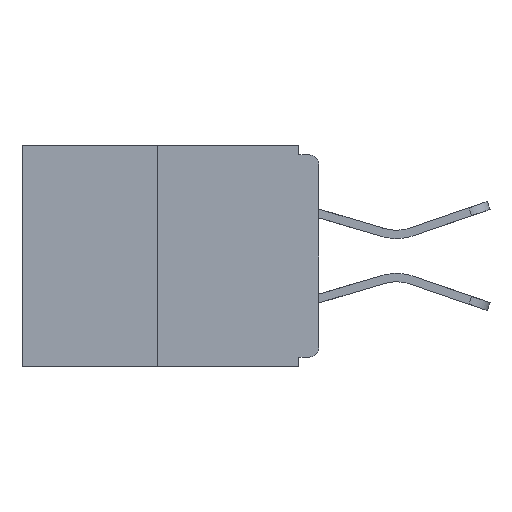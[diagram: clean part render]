
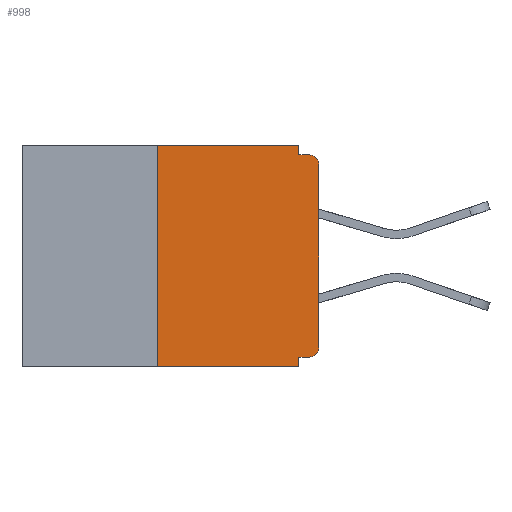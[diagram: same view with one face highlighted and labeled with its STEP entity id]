
A CAD part, left-side view. The second image highlights one B-rep face of the part: STEP entity #998.
In plain terms, the highlighted planar face has unit normal (-1, 0, 0).
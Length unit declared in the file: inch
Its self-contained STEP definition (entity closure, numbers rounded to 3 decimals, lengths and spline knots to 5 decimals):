
#89 = DIRECTION ( 'NONE',  ( 1., 0., 0. ) ) ;
#129 = DIRECTION ( 'NONE',  ( -1., 0., 0. ) ) ;
#150 = VERTEX_POINT ( 'NONE', #5514 ) ;
#182 = VECTOR ( 'NONE', #2445, 39.37008 ) ;
#286 = EDGE_CURVE ( 'NONE', #150, #296, #9862, .T. ) ;
#296 = VERTEX_POINT ( 'NONE', #3870 ) ;
#387 = AXIS2_PLACEMENT_3D ( 'NONE', #6551, #129, #1014 ) ;
#467 = CARTESIAN_POINT ( 'NONE',  ( 0., 0.031, -0.015 ) ) ;
#834 = ORIENTED_EDGE ( 'NONE', *, *, #11553, .T. ) ;
#934 = CARTESIAN_POINT ( 'NONE',  ( 0., 0., -0.015 ) ) ;
#998 = ADVANCED_FACE ( 'NONE', ( #4077 ), #4645, .F. ) ;
#1014 = DIRECTION ( 'NONE',  ( 0., 0., -1. ) ) ;
#1047 = LINE ( 'NONE', #1260, #4214 ) ;
#1260 = CARTESIAN_POINT ( 'NONE',  ( 0., 0., -0.328 ) ) ;
#1439 = DIRECTION ( 'NONE',  ( 0., -1., 0. ) ) ;
#1524 = CARTESIAN_POINT ( 'NONE',  ( 0., 0.25, 0. ) ) ;
#1578 = DIRECTION ( 'NONE',  ( 0., -1., 0. ) ) ;
#1853 = VERTEX_POINT ( 'NONE', #8227 ) ;
#2208 = LINE ( 'NONE', #5937, #7402 ) ;
#2445 = DIRECTION ( 'NONE',  ( 0., 0., 1. ) ) ;
#2594 = AXIS2_PLACEMENT_3D ( 'NONE', #10205, #89, #6673 ) ;
#2837 = ORIENTED_EDGE ( 'NONE', *, *, #9714, .T. ) ;
#3101 = EDGE_CURVE ( 'NONE', #1853, #10226, #9412, .T. ) ;
#3287 = DIRECTION ( 'NONE',  ( 0., 0., -1. ) ) ;
#3870 = CARTESIAN_POINT ( 'NONE',  ( 0., 0.031, -0.343 ) ) ;
#3915 = CARTESIAN_POINT ( 'NONE',  ( 0., 0., -0.313 ) ) ;
#3961 = CARTESIAN_POINT ( 'NONE',  ( 0., 0.015, -0.328 ) ) ;
#4077 = FACE_OUTER_BOUND ( 'NONE', #4302, .T. ) ;
#4214 = VECTOR ( 'NONE', #10363, 39.37008 ) ;
#4229 = DIRECTION ( 'NONE',  ( 0., 0., -1. ) ) ;
#4302 = EDGE_LOOP ( 'NONE', ( #8157, #7699, #10369, #8915, #7518, #834, #2837, #8779, #9005, #10305 ) ) ;
#4442 = CARTESIAN_POINT ( 'NONE',  ( 0., 0., -0.03 ) ) ;
#4645 = PLANE ( 'NONE',  #2594 ) ;
#4721 = EDGE_CURVE ( 'NONE', #1853, #296, #9951, .T. ) ;
#4926 = VERTEX_POINT ( 'NONE', #3961 ) ;
#4972 = AXIS2_PLACEMENT_3D ( 'NONE', #11584, #9837, #3287 ) ;
#5293 = CARTESIAN_POINT ( 'NONE',  ( 0., 0.46, -0.343 ) ) ;
#5315 = EDGE_CURVE ( 'NONE', #11823, #6057, #11917, .T. ) ;
#5514 = CARTESIAN_POINT ( 'NONE',  ( 0., 0.031, -0.328 ) ) ;
#5564 = CARTESIAN_POINT ( 'NONE',  ( 0., 0.015, -0.015 ) ) ;
#5712 = CARTESIAN_POINT ( 'NONE',  ( 0., 0., 0. ) ) ;
#5937 = CARTESIAN_POINT ( 'NONE',  ( 0., 0.031, 0. ) ) ;
#6057 = VERTEX_POINT ( 'NONE', #5564 ) ;
#6310 = EDGE_CURVE ( 'NONE', #11506, #6057, #7769, .T. ) ;
#6551 = CARTESIAN_POINT ( 'NONE',  ( 0., 0.015, -0.313 ) ) ;
#6673 = DIRECTION ( 'NONE',  ( 0., 0., -1. ) ) ;
#7171 = CARTESIAN_POINT ( 'NONE',  ( 0., 0.031, -0.343 ) ) ;
#7391 = DIRECTION ( 'NONE',  ( 0., -1., 0. ) ) ;
#7402 = VECTOR ( 'NONE', #4229, 39.37008 ) ;
#7415 = VECTOR ( 'NONE', #9411, 39.37008 ) ;
#7518 = ORIENTED_EDGE ( 'NONE', *, *, #11753, .F. ) ;
#7652 = VECTOR ( 'NONE', #7391, 39.37008 ) ;
#7699 = ORIENTED_EDGE ( 'NONE', *, *, #3101, .F. ) ;
#7716 = CIRCLE ( 'NONE', #387, 0.015 ) ;
#7723 = DIRECTION ( 'NONE',  ( 0., 0., 1. ) ) ;
#7769 = CIRCLE ( 'NONE', #4972, 0.015 ) ;
#7846 = EDGE_CURVE ( 'NONE', #10226, #11395, #10869, .T. ) ;
#7945 = CARTESIAN_POINT ( 'NONE',  ( 0., 0.46, 0. ) ) ;
#8157 = ORIENTED_EDGE ( 'NONE', *, *, #7846, .F. ) ;
#8227 = CARTESIAN_POINT ( 'NONE',  ( 0., 0.25, -0.343 ) ) ;
#8779 = ORIENTED_EDGE ( 'NONE', *, *, #6310, .T. ) ;
#8915 = ORIENTED_EDGE ( 'NONE', *, *, #286, .F. ) ;
#9005 = ORIENTED_EDGE ( 'NONE', *, *, #5315, .F. ) ;
#9326 = LINE ( 'NONE', #5712, #11894 ) ;
#9411 = DIRECTION ( 'NONE',  ( 0., 0., -1. ) ) ;
#9412 = LINE ( 'NONE', #1524, #182 ) ;
#9464 = CARTESIAN_POINT ( 'NONE',  ( 0., 0.25, 0. ) ) ;
#9714 = EDGE_CURVE ( 'NONE', #11735, #11506, #9326, .T. ) ;
#9837 = DIRECTION ( 'NONE',  ( -1., 0., 0. ) ) ;
#9862 = LINE ( 'NONE', #7171, #7415 ) ;
#9951 = LINE ( 'NONE', #5293, #10798 ) ;
#9963 = CARTESIAN_POINT ( 'NONE',  ( 0., 0.031, 0. ) ) ;
#10205 = CARTESIAN_POINT ( 'NONE',  ( 0., 0.46, 0. ) ) ;
#10226 = VERTEX_POINT ( 'NONE', #9464 ) ;
#10305 = ORIENTED_EDGE ( 'NONE', *, *, #11803, .F. ) ;
#10363 = DIRECTION ( 'NONE',  ( 0., 1., 0. ) ) ;
#10369 = ORIENTED_EDGE ( 'NONE', *, *, #4721, .T. ) ;
#10721 = VECTOR ( 'NONE', #1439, 39.37008 ) ;
#10798 = VECTOR ( 'NONE', #1578, 39.37008 ) ;
#10869 = LINE ( 'NONE', #7945, #10721 ) ;
#11395 = VERTEX_POINT ( 'NONE', #9963 ) ;
#11506 = VERTEX_POINT ( 'NONE', #4442 ) ;
#11553 = EDGE_CURVE ( 'NONE', #4926, #11735, #7716, .T. ) ;
#11584 = CARTESIAN_POINT ( 'NONE',  ( 0., 0.015, -0.03 ) ) ;
#11735 = VERTEX_POINT ( 'NONE', #3915 ) ;
#11753 = EDGE_CURVE ( 'NONE', #4926, #150, #1047, .T. ) ;
#11803 = EDGE_CURVE ( 'NONE', #11395, #11823, #2208, .T. ) ;
#11823 = VERTEX_POINT ( 'NONE', #467 ) ;
#11894 = VECTOR ( 'NONE', #7723, 39.37008 ) ;
#11917 = LINE ( 'NONE', #934, #7652 ) ;
